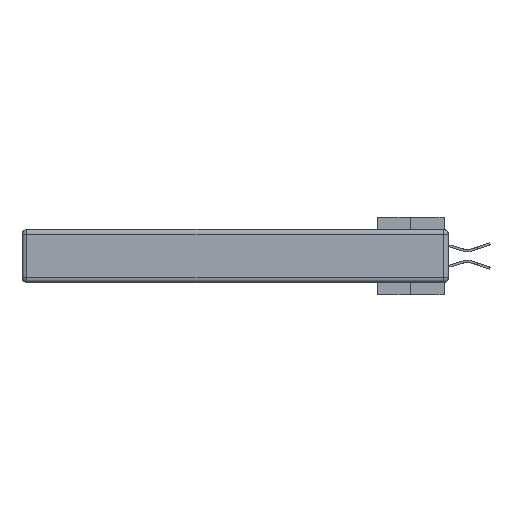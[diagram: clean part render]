
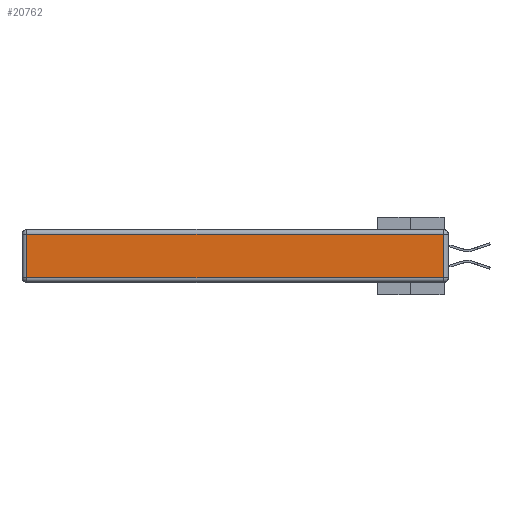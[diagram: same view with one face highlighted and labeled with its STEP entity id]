
A CAD part, left-side view. The second image highlights one B-rep face of the part: STEP entity #20762.
In plain terms, the highlighted planar face has unit normal (-1, 0, 0).
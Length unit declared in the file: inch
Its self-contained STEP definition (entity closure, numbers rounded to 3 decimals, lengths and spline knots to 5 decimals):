
#580 = CARTESIAN_POINT ( 'NONE',  ( 0., 0.03, -0.03 ) ) ;
#608 = VERTEX_POINT ( 'NONE', #3006 ) ;
#875 = VERTEX_POINT ( 'NONE', #5013 ) ;
#1066 = CARTESIAN_POINT ( 'NONE',  ( 0., 0.03, -0.343 ) ) ;
#1210 = AXIS2_PLACEMENT_3D ( 'NONE', #19399, #12949, #6396 ) ;
#2749 = VECTOR ( 'NONE', #25957, 39.37008 ) ;
#3006 = CARTESIAN_POINT ( 'NONE',  ( 0., 0.03, -0.313 ) ) ;
#5013 = CARTESIAN_POINT ( 'NONE',  ( 0., 2.72, -0.313 ) ) ;
#6004 = EDGE_LOOP ( 'NONE', ( #14684, #16897, #8172, #34044 ) ) ;
#6254 = VECTOR ( 'NONE', #13166, 39.37008 ) ;
#6305 = LINE ( 'NONE', #40391, #6254 ) ;
#6396 = DIRECTION ( 'NONE',  ( 0., 0., 1. ) ) ;
#6540 = EDGE_CURVE ( 'NONE', #608, #30930, #34248, .T. ) ;
#6711 = EDGE_CURVE ( 'NONE', #30930, #24465, #6305, .T. ) ;
#8172 = ORIENTED_EDGE ( 'NONE', *, *, #6711, .T. ) ;
#8457 = LINE ( 'NONE', #22594, #2749 ) ;
#12350 = VECTOR ( 'NONE', #14319, 39.37008 ) ;
#12949 = DIRECTION ( 'NONE',  ( -1., 0., 0. ) ) ;
#13166 = DIRECTION ( 'NONE',  ( 0., 1., 0. ) ) ;
#13775 = LINE ( 'NONE', #32274, #32510 ) ;
#14319 = DIRECTION ( 'NONE',  ( 0., 0., 1. ) ) ;
#14684 = ORIENTED_EDGE ( 'NONE', *, *, #39366, .T. ) ;
#16897 = ORIENTED_EDGE ( 'NONE', *, *, #6540, .T. ) ;
#19399 = CARTESIAN_POINT ( 'NONE',  ( 0., 0., -0.343 ) ) ;
#19662 = PLANE ( 'NONE',  #1210 ) ;
#20762 = ADVANCED_FACE ( 'NONE', ( #24488 ), #19662, .T. ) ;
#22594 = CARTESIAN_POINT ( 'NONE',  ( 0., 0., -0.313 ) ) ;
#24465 = VERTEX_POINT ( 'NONE', #35299 ) ;
#24488 = FACE_OUTER_BOUND ( 'NONE', #6004, .T. ) ;
#25957 = DIRECTION ( 'NONE',  ( 0., -1., 0. ) ) ;
#29222 = EDGE_CURVE ( 'NONE', #24465, #875, #13775, .T. ) ;
#30930 = VERTEX_POINT ( 'NONE', #580 ) ;
#32274 = CARTESIAN_POINT ( 'NONE',  ( 0., 2.72, -0.343 ) ) ;
#32510 = VECTOR ( 'NONE', #35634, 39.37008 ) ;
#34044 = ORIENTED_EDGE ( 'NONE', *, *, #29222, .T. ) ;
#34248 = LINE ( 'NONE', #1066, #12350 ) ;
#35299 = CARTESIAN_POINT ( 'NONE',  ( 0., 2.72, -0.03 ) ) ;
#35634 = DIRECTION ( 'NONE',  ( 0., 0., -1. ) ) ;
#39366 = EDGE_CURVE ( 'NONE', #875, #608, #8457, .T. ) ;
#40391 = CARTESIAN_POINT ( 'NONE',  ( 0., 2.75, -0.03 ) ) ;
